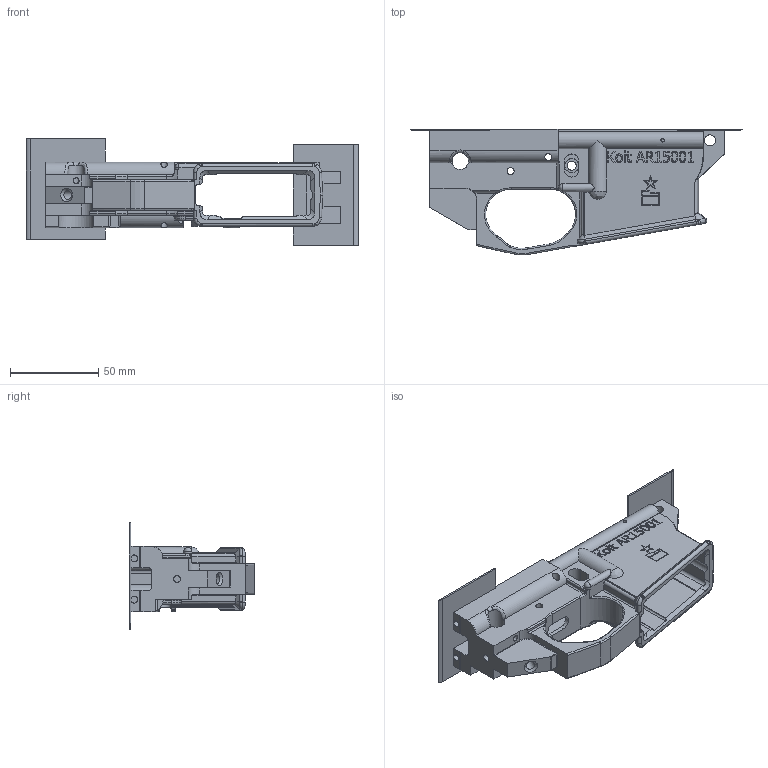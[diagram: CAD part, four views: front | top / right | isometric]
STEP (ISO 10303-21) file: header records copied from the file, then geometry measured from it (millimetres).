
FILE_DESCRIPTION(/* description */ (' '),/* implementation_level */ '2;1');
FILE_NAME(/* name */ 'Lower Body.stp',/* time_stamp */ '2019-07-22T21:10:50-05:00',/* author */ ('johne'),/* organization */ (' '),/* preprocessor_version */ 'ST-DEVELOPER v16.13',/* originating_system */ 'Autodesk Inventor 2018',/* authorisation */ ' ');
FILE_SCHEMA (('AUTOMOTIVE_DESIGN { 1 0 10303 214 3 1 1 }'));
Length unit declared in the file: inch
Products named in the file (1): Lower Body
Bounding box: 188.05 x 71.27 x 60.34 mm (x, y, z)
Volume: 105564.9 mm3; surface area: 57418.3 mm2
Topology: 1 solids, 1 shells, 1157 faces, 3145 edges, 2051 vertices
Faces by surface type: plane 683, bspline 248, cylinder 179, torus 37, sphere 7, cone 3
Full cylindrical faces by diameter (mm): 1.981 x1, 2.362 x2, 2.464 x1, 3.175 x1, 3.937 x1, 3.969 x5, 5.105 x1, 5.182 x1, 6.375 x2, 7.938 x1, 9.525 x2
Entity records: 43152 total; most frequent: CARTESIAN_POINT 15537, ORIENTED_EDGE 6216, DIRECTION 4771, EDGE_CURVE 3108, LINE 2167, VECTOR 2167, VERTEX_POINT 2042, AXIS2_PLACEMENT_3D 1302
